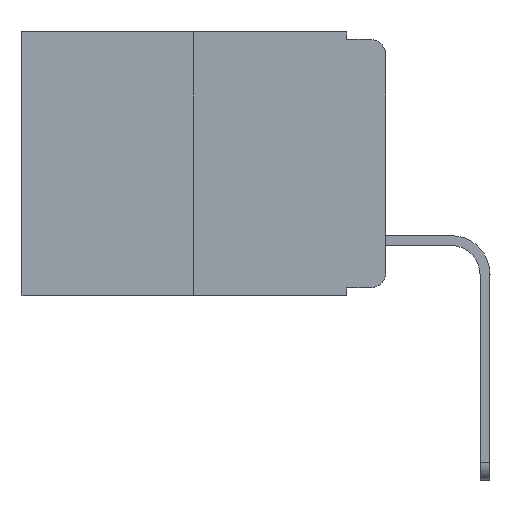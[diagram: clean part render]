
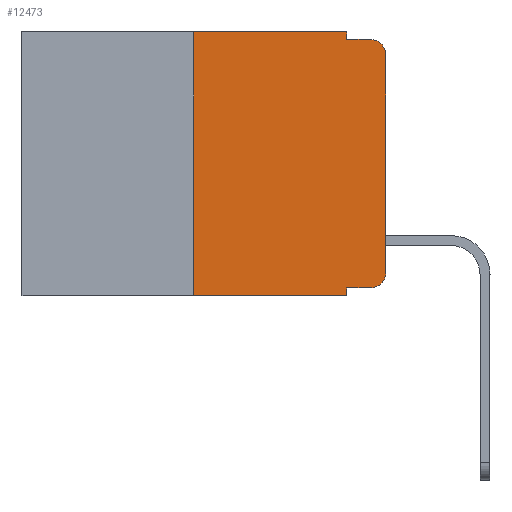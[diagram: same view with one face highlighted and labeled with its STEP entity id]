
A CAD part, left-side view. The second image highlights one B-rep face of the part: STEP entity #12473.
In plain terms, the highlighted planar face has unit normal (-1, 0, 0).
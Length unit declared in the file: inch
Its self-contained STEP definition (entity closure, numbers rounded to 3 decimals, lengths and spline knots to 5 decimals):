
#89 = CARTESIAN_POINT ( 'NONE',  ( 0., 0., -0.03 ) ) ;
#287 = VECTOR ( 'NONE', #19640, 39.37008 ) ;
#1359 = DIRECTION ( 'NONE',  ( 0., 0., 1. ) ) ;
#1425 = CARTESIAN_POINT ( 'NONE',  ( 0., 0.051, -0.01 ) ) ;
#1428 = FACE_OUTER_BOUND ( 'NONE', #14472, .T. ) ;
#1653 = CARTESIAN_POINT ( 'NONE',  ( 0., 0.02, -0.313 ) ) ;
#1965 = DIRECTION ( 'NONE',  ( -1., 0., 0. ) ) ;
#2171 = VECTOR ( 'NONE', #3174, 39.37008 ) ;
#2472 = EDGE_CURVE ( 'NONE', #20216, #6268, #15321, .T. ) ;
#2785 = DIRECTION ( 'NONE',  ( 0., 0., -1. ) ) ;
#2910 = EDGE_CURVE ( 'NONE', #17548, #17217, #14278, .T. ) ;
#3174 = DIRECTION ( 'NONE',  ( 0., -1., 0. ) ) ;
#3692 = LINE ( 'NONE', #11082, #4691 ) ;
#3923 = LINE ( 'NONE', #1425, #2171 ) ;
#4691 = VECTOR ( 'NONE', #1359, 39.37008 ) ;
#4717 = ORIENTED_EDGE ( 'NONE', *, *, #14968, .F. ) ;
#5518 = CARTESIAN_POINT ( 'NONE',  ( 0., 0.051, -0.01 ) ) ;
#5836 = ORIENTED_EDGE ( 'NONE', *, *, #13549, .T. ) ;
#6100 = DIRECTION ( 'NONE',  ( 0., 0., -1. ) ) ;
#6268 = VERTEX_POINT ( 'NONE', #18550 ) ;
#6297 = CARTESIAN_POINT ( 'NONE',  ( 0., 0.051, -0.343 ) ) ;
#6656 = EDGE_CURVE ( 'NONE', #18078, #7874, #12970, .T. ) ;
#7019 = VERTEX_POINT ( 'NONE', #19199 ) ;
#7408 = DIRECTION ( 'NONE',  ( 0., -1., 0. ) ) ;
#7435 = DIRECTION ( 'NONE',  ( 0., 0., 1. ) ) ;
#7874 = VERTEX_POINT ( 'NONE', #6297 ) ;
#8739 = VECTOR ( 'NONE', #14076, 39.37008 ) ;
#8857 = VECTOR ( 'NONE', #15209, 39.37008 ) ;
#8871 = EDGE_CURVE ( 'NONE', #7019, #16025, #17178, .T. ) ;
#8997 = VECTOR ( 'NONE', #7435, 39.37008 ) ;
#9202 = EDGE_CURVE ( 'NONE', #16025, #20216, #14218, .T. ) ;
#9470 = DIRECTION ( 'NONE',  ( 1., 0., 0. ) ) ;
#9551 = CARTESIAN_POINT ( 'NONE',  ( 0., 0.473, 0. ) ) ;
#9979 = EDGE_CURVE ( 'NONE', #17238, #17548, #3692, .T. ) ;
#9996 = DIRECTION ( 'NONE',  ( 0., 0., -1. ) ) ;
#10717 = CARTESIAN_POINT ( 'NONE',  ( 0., 0.051, 0. ) ) ;
#10729 = EDGE_CURVE ( 'NONE', #19558, #6268, #3923, .T. ) ;
#11082 = CARTESIAN_POINT ( 'NONE',  ( 0., 0.25, 0. ) ) ;
#11307 = CARTESIAN_POINT ( 'NONE',  ( 0., 0.02, -0.03 ) ) ;
#11325 = CARTESIAN_POINT ( 'NONE',  ( 0., 0.473, 0. ) ) ;
#12232 = CARTESIAN_POINT ( 'NONE',  ( 0., 0., 0. ) ) ;
#12473 = ADVANCED_FACE ( 'NONE', ( #1428 ), #15640, .F. ) ;
#12970 = LINE ( 'NONE', #13440, #287 ) ;
#13341 = AXIS2_PLACEMENT_3D ( 'NONE', #1653, #18706, #2785 ) ;
#13390 = CARTESIAN_POINT ( 'NONE',  ( 0., 0., -0.313 ) ) ;
#13440 = CARTESIAN_POINT ( 'NONE',  ( 0., 0.051, 0. ) ) ;
#13549 = EDGE_CURVE ( 'NONE', #18078, #7019, #19346, .T. ) ;
#13550 = CARTESIAN_POINT ( 'NONE',  ( 0., 0.051, -0.333 ) ) ;
#13723 = CARTESIAN_POINT ( 'NONE',  ( 0., 0.25, -0.343 ) ) ;
#13994 = CARTESIAN_POINT ( 'NONE',  ( 0., 0.051, 0. ) ) ;
#14076 = DIRECTION ( 'NONE',  ( 0., 0., -1. ) ) ;
#14218 = LINE ( 'NONE', #12232, #8997 ) ;
#14260 = ORIENTED_EDGE ( 'NONE', *, *, #19863, .T. ) ;
#14278 = LINE ( 'NONE', #11325, #16827 ) ;
#14472 = EDGE_LOOP ( 'NONE', ( #18080, #14786, #15051, #4717, #19650, #16245, #14260, #15199, #5836, #18282 ) ) ;
#14786 = ORIENTED_EDGE ( 'NONE', *, *, #2472, .T. ) ;
#14968 = EDGE_CURVE ( 'NONE', #17217, #19558, #19257, .T. ) ;
#15051 = ORIENTED_EDGE ( 'NONE', *, *, #10729, .F. ) ;
#15199 = ORIENTED_EDGE ( 'NONE', *, *, #6656, .F. ) ;
#15209 = DIRECTION ( 'NONE',  ( 0., -1., 0. ) ) ;
#15321 = CIRCLE ( 'NONE', #17684, 0.02 ) ;
#15640 = PLANE ( 'NONE',  #19978 ) ;
#16025 = VERTEX_POINT ( 'NONE', #13390 ) ;
#16245 = ORIENTED_EDGE ( 'NONE', *, *, #9979, .F. ) ;
#16827 = VECTOR ( 'NONE', #17804, 39.37008 ) ;
#16908 = CARTESIAN_POINT ( 'NONE',  ( 0., 0.473, -0.343 ) ) ;
#17178 = CIRCLE ( 'NONE', #13341, 0.02 ) ;
#17217 = VERTEX_POINT ( 'NONE', #10717 ) ;
#17238 = VERTEX_POINT ( 'NONE', #13723 ) ;
#17548 = VERTEX_POINT ( 'NONE', #17883 ) ;
#17648 = CARTESIAN_POINT ( 'NONE',  ( 0., 0.051, -0.333 ) ) ;
#17684 = AXIS2_PLACEMENT_3D ( 'NONE', #11307, #1965, #9996 ) ;
#17804 = DIRECTION ( 'NONE',  ( 0., -1., 0. ) ) ;
#17883 = CARTESIAN_POINT ( 'NONE',  ( 0., 0.25, 0. ) ) ;
#18078 = VERTEX_POINT ( 'NONE', #17648 ) ;
#18080 = ORIENTED_EDGE ( 'NONE', *, *, #9202, .T. ) ;
#18106 = LINE ( 'NONE', #16908, #8857 ) ;
#18282 = ORIENTED_EDGE ( 'NONE', *, *, #8871, .T. ) ;
#18550 = CARTESIAN_POINT ( 'NONE',  ( 0., 0.02, -0.01 ) ) ;
#18706 = DIRECTION ( 'NONE',  ( -1., 0., 0. ) ) ;
#18837 = VECTOR ( 'NONE', #7408, 39.37008 ) ;
#19199 = CARTESIAN_POINT ( 'NONE',  ( 0., 0.02, -0.333 ) ) ;
#19257 = LINE ( 'NONE', #13994, #8739 ) ;
#19346 = LINE ( 'NONE', #13550, #18837 ) ;
#19558 = VERTEX_POINT ( 'NONE', #5518 ) ;
#19640 = DIRECTION ( 'NONE',  ( 0., 0., -1. ) ) ;
#19650 = ORIENTED_EDGE ( 'NONE', *, *, #2910, .F. ) ;
#19863 = EDGE_CURVE ( 'NONE', #17238, #7874, #18106, .T. ) ;
#19978 = AXIS2_PLACEMENT_3D ( 'NONE', #9551, #9470, #6100 ) ;
#20216 = VERTEX_POINT ( 'NONE', #89 ) ;
